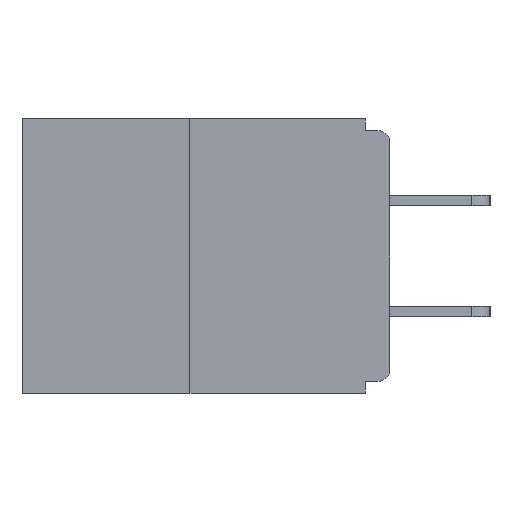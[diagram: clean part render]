
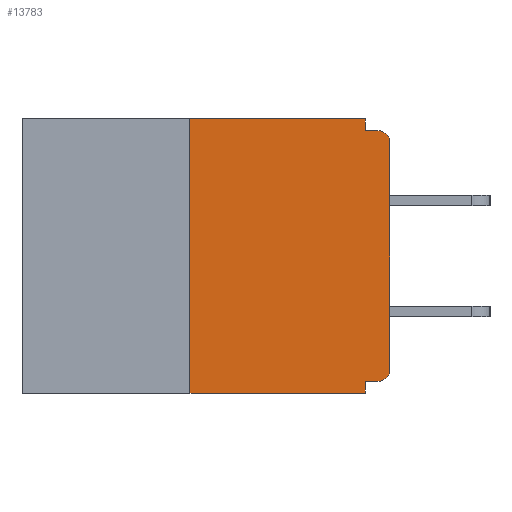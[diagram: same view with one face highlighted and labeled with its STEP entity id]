
A CAD part, left-side view. The second image highlights one B-rep face of the part: STEP entity #13783.
In plain terms, the highlighted planar face has unit normal (-1, 0, 0).
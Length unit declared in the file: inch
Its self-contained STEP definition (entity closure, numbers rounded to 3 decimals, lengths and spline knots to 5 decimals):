
#150 = LINE ( 'NONE', #11938, #9127 ) ;
#176 = CARTESIAN_POINT ( 'NONE',  ( 0., 0.46, -0.343 ) ) ;
#562 = AXIS2_PLACEMENT_3D ( 'NONE', #2053, #15383, #14167 ) ;
#863 = CARTESIAN_POINT ( 'NONE',  ( 0., 0.46, 0. ) ) ;
#1028 = ORIENTED_EDGE ( 'NONE', *, *, #1782, .T. ) ;
#1330 = VECTOR ( 'NONE', #17537, 39.37008 ) ;
#1400 = LINE ( 'NONE', #19795, #16962 ) ;
#1567 = ORIENTED_EDGE ( 'NONE', *, *, #12175, .F. ) ;
#1782 = EDGE_CURVE ( 'NONE', #19760, #8452, #18610, .T. ) ;
#2053 = CARTESIAN_POINT ( 'NONE',  ( 0., 0.015, -0.03 ) ) ;
#2148 = EDGE_CURVE ( 'NONE', #3610, #18173, #10303, .T. ) ;
#2941 = DIRECTION ( 'NONE',  ( 0., 0., 1. ) ) ;
#3072 = VECTOR ( 'NONE', #6885, 39.37008 ) ;
#3130 = EDGE_CURVE ( 'NONE', #8452, #3243, #150, .T. ) ;
#3243 = VERTEX_POINT ( 'NONE', #20638 ) ;
#3407 = ORIENTED_EDGE ( 'NONE', *, *, #7380, .F. ) ;
#3610 = VERTEX_POINT ( 'NONE', #13982 ) ;
#3780 = DIRECTION ( 'NONE',  ( 0., -1., 0. ) ) ;
#4374 = VERTEX_POINT ( 'NONE', #7081 ) ;
#4457 = VECTOR ( 'NONE', #13913, 39.37008 ) ;
#4510 = ORIENTED_EDGE ( 'NONE', *, *, #10406, .F. ) ;
#5038 = CARTESIAN_POINT ( 'NONE',  ( 0., 0.031, 0. ) ) ;
#5495 = EDGE_CURVE ( 'NONE', #20394, #16127, #12147, .T. ) ;
#5650 = CARTESIAN_POINT ( 'NONE',  ( 0., 0.46, 0. ) ) ;
#5735 = CARTESIAN_POINT ( 'NONE',  ( 0., 0.015, -0.328 ) ) ;
#6152 = CARTESIAN_POINT ( 'NONE',  ( 0., 0., -0.328 ) ) ;
#6584 = VECTOR ( 'NONE', #3780, 39.37008 ) ;
#6641 = CARTESIAN_POINT ( 'NONE',  ( 0., 0.25, 0. ) ) ;
#6751 = LINE ( 'NONE', #13485, #6584 ) ;
#6885 = DIRECTION ( 'NONE',  ( 0., -1., 0. ) ) ;
#6910 = ORIENTED_EDGE ( 'NONE', *, *, #3130, .T. ) ;
#7081 = CARTESIAN_POINT ( 'NONE',  ( 0., 0.031, -0.328 ) ) ;
#7154 = LINE ( 'NONE', #7266, #20803 ) ;
#7266 = CARTESIAN_POINT ( 'NONE',  ( 0., 0.031, -0.343 ) ) ;
#7380 = EDGE_CURVE ( 'NONE', #4374, #18173, #7154, .T. ) ;
#7434 = VERTEX_POINT ( 'NONE', #20723 ) ;
#7680 = DIRECTION ( 'NONE',  ( 1., 0., 0. ) ) ;
#8184 = ORIENTED_EDGE ( 'NONE', *, *, #8798, .F. ) ;
#8452 = VERTEX_POINT ( 'NONE', #9718 ) ;
#8798 = EDGE_CURVE ( 'NONE', #3610, #20394, #1400, .T. ) ;
#8810 = DIRECTION ( 'NONE',  ( -1., 0., 0. ) ) ;
#9127 = VECTOR ( 'NONE', #18655, 39.37008 ) ;
#9277 = CARTESIAN_POINT ( 'NONE',  ( 0., 0.031, -0.343 ) ) ;
#9718 = CARTESIAN_POINT ( 'NONE',  ( 0., 0., -0.313 ) ) ;
#10303 = LINE ( 'NONE', #176, #3072 ) ;
#10406 = EDGE_CURVE ( 'NONE', #7434, #18260, #6751, .T. ) ;
#10568 = ORIENTED_EDGE ( 'NONE', *, *, #17555, .T. ) ;
#11938 = CARTESIAN_POINT ( 'NONE',  ( 0., 0., 0. ) ) ;
#12147 = LINE ( 'NONE', #5650, #13227 ) ;
#12175 = EDGE_CURVE ( 'NONE', #19760, #4374, #19599, .T. ) ;
#12281 = EDGE_LOOP ( 'NONE', ( #21570, #8184, #19563, #3407, #1567, #1028, #6910, #10568, #4510, #17991 ) ) ;
#12689 = AXIS2_PLACEMENT_3D ( 'NONE', #17405, #8810, #17302 ) ;
#13227 = VECTOR ( 'NONE', #13700, 39.37008 ) ;
#13485 = CARTESIAN_POINT ( 'NONE',  ( 0., 0., -0.015 ) ) ;
#13700 = DIRECTION ( 'NONE',  ( 0., -1., 0. ) ) ;
#13783 = ADVANCED_FACE ( 'NONE', ( #17274 ), #15845, .F. ) ;
#13913 = DIRECTION ( 'NONE',  ( 0., 0., -1. ) ) ;
#13982 = CARTESIAN_POINT ( 'NONE',  ( 0., 0.25, -0.343 ) ) ;
#14167 = DIRECTION ( 'NONE',  ( 0., 0., -1. ) ) ;
#14863 = AXIS2_PLACEMENT_3D ( 'NONE', #863, #7680, #20808 ) ;
#15383 = DIRECTION ( 'NONE',  ( -1., 0., 0. ) ) ;
#15678 = LINE ( 'NONE', #18865, #4457 ) ;
#15845 = PLANE ( 'NONE',  #14863 ) ;
#16127 = VERTEX_POINT ( 'NONE', #5038 ) ;
#16861 = CARTESIAN_POINT ( 'NONE',  ( 0., 0.015, -0.015 ) ) ;
#16962 = VECTOR ( 'NONE', #2941, 39.37008 ) ;
#17274 = FACE_OUTER_BOUND ( 'NONE', #12281, .T. ) ;
#17302 = DIRECTION ( 'NONE',  ( 0., 0., -1. ) ) ;
#17405 = CARTESIAN_POINT ( 'NONE',  ( 0., 0.015, -0.313 ) ) ;
#17537 = DIRECTION ( 'NONE',  ( 0., 1., 0. ) ) ;
#17555 = EDGE_CURVE ( 'NONE', #3243, #18260, #18155, .T. ) ;
#17910 = EDGE_CURVE ( 'NONE', #16127, #7434, #15678, .T. ) ;
#17991 = ORIENTED_EDGE ( 'NONE', *, *, #17910, .F. ) ;
#18155 = CIRCLE ( 'NONE', #562, 0.015 ) ;
#18173 = VERTEX_POINT ( 'NONE', #9277 ) ;
#18260 = VERTEX_POINT ( 'NONE', #16861 ) ;
#18610 = CIRCLE ( 'NONE', #12689, 0.015 ) ;
#18655 = DIRECTION ( 'NONE',  ( 0., 0., 1. ) ) ;
#18865 = CARTESIAN_POINT ( 'NONE',  ( 0., 0.031, 0. ) ) ;
#19563 = ORIENTED_EDGE ( 'NONE', *, *, #2148, .T. ) ;
#19599 = LINE ( 'NONE', #6152, #1330 ) ;
#19760 = VERTEX_POINT ( 'NONE', #5735 ) ;
#19795 = CARTESIAN_POINT ( 'NONE',  ( 0., 0.25, 0. ) ) ;
#20394 = VERTEX_POINT ( 'NONE', #6641 ) ;
#20604 = DIRECTION ( 'NONE',  ( 0., 0., -1. ) ) ;
#20638 = CARTESIAN_POINT ( 'NONE',  ( 0., 0., -0.03 ) ) ;
#20723 = CARTESIAN_POINT ( 'NONE',  ( 0., 0.031, -0.015 ) ) ;
#20803 = VECTOR ( 'NONE', #20604, 39.37008 ) ;
#20808 = DIRECTION ( 'NONE',  ( 0., 0., -1. ) ) ;
#21570 = ORIENTED_EDGE ( 'NONE', *, *, #5495, .F. ) ;
